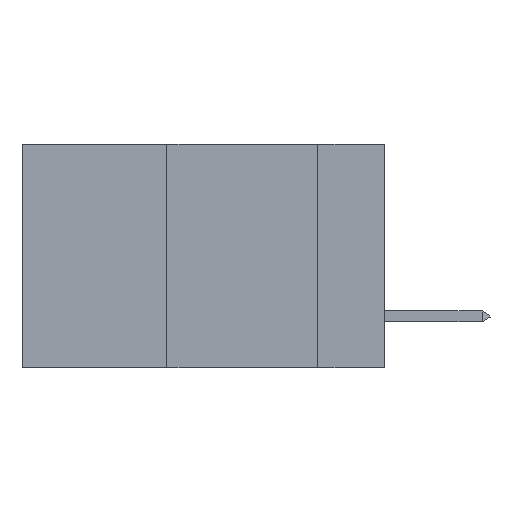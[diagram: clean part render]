
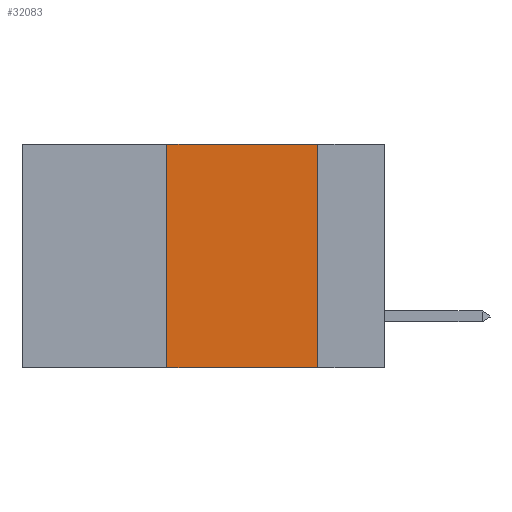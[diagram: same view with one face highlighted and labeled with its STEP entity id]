
A CAD part, left-side view. The second image highlights one B-rep face of the part: STEP entity #32083.
In plain terms, the highlighted planar face has unit normal (-1, 0, 0).
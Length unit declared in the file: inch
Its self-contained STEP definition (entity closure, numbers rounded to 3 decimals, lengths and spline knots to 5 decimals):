
#1962 = ORIENTED_EDGE ( 'NONE', *, *, #3852, .F. ) ;
#2501 = LINE ( 'NONE', #13653, #16370 ) ;
#2601 = CARTESIAN_POINT ( 'NONE',  ( 0., 0.11, -0.37 ) ) ;
#3852 = EDGE_CURVE ( 'NONE', #12856, #33141, #21400, .T. ) ;
#3874 = ORIENTED_EDGE ( 'NONE', *, *, #24937, .F. ) ;
#3954 = DIRECTION ( 'NONE',  ( 0., -1., 0. ) ) ;
#6297 = PLANE ( 'NONE',  #34300 ) ;
#7097 = VECTOR ( 'NONE', #34815, 39.37008 ) ;
#7881 = ORIENTED_EDGE ( 'NONE', *, *, #9019, .F. ) ;
#9019 = EDGE_CURVE ( 'NONE', #34271, #20369, #2501, .T. ) ;
#10595 = CARTESIAN_POINT ( 'NONE',  ( 0., 0.36, 0. ) ) ;
#11556 = VECTOR ( 'NONE', #3954, 39.37008 ) ;
#11668 = CARTESIAN_POINT ( 'NONE',  ( 0., 0.6, 0. ) ) ;
#11825 = CARTESIAN_POINT ( 'NONE',  ( 0., 0.6, -0.37 ) ) ;
#12856 = VERTEX_POINT ( 'NONE', #32000 ) ;
#12926 = FACE_OUTER_BOUND ( 'NONE', #17910, .T. ) ;
#13284 = DIRECTION ( 'NONE',  ( 0., -1., 0. ) ) ;
#13653 = CARTESIAN_POINT ( 'NONE',  ( 0., 0.11, 0. ) ) ;
#16328 = CARTESIAN_POINT ( 'NONE',  ( 0., 0.6, 0. ) ) ;
#16362 = DIRECTION ( 'NONE',  ( 0., 0., -1. ) ) ;
#16370 = VECTOR ( 'NONE', #16362, 39.37008 ) ;
#16609 = LINE ( 'NONE', #11825, #11556 ) ;
#17089 = DIRECTION ( 'NONE',  ( 1., 0., 0. ) ) ;
#17910 = EDGE_LOOP ( 'NONE', ( #7881, #3874, #1962, #32542 ) ) ;
#20369 = VERTEX_POINT ( 'NONE', #2601 ) ;
#21400 = LINE ( 'NONE', #10595, #7097 ) ;
#21624 = LINE ( 'NONE', #16328, #29619 ) ;
#24521 = EDGE_CURVE ( 'NONE', #12856, #20369, #16609, .T. ) ;
#24937 = EDGE_CURVE ( 'NONE', #33141, #34271, #21624, .T. ) ;
#25330 = DIRECTION ( 'NONE',  ( 0., 0., -1. ) ) ;
#29619 = VECTOR ( 'NONE', #13284, 39.37008 ) ;
#30130 = CARTESIAN_POINT ( 'NONE',  ( 0., 0.36, 0. ) ) ;
#32000 = CARTESIAN_POINT ( 'NONE',  ( 0., 0.36, -0.37 ) ) ;
#32083 = ADVANCED_FACE ( 'NONE', ( #12926 ), #6297, .F. ) ;
#32542 = ORIENTED_EDGE ( 'NONE', *, *, #24521, .T. ) ;
#33141 = VERTEX_POINT ( 'NONE', #30130 ) ;
#34271 = VERTEX_POINT ( 'NONE', #34393 ) ;
#34300 = AXIS2_PLACEMENT_3D ( 'NONE', #11668, #17089, #25330 ) ;
#34393 = CARTESIAN_POINT ( 'NONE',  ( 0., 0.11, 0. ) ) ;
#34815 = DIRECTION ( 'NONE',  ( 0., 0., 1. ) ) ;
